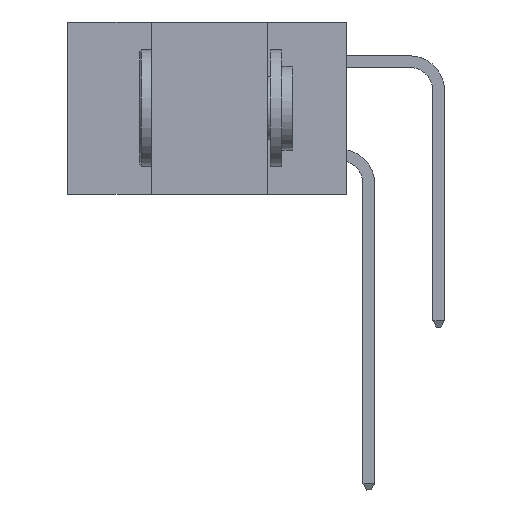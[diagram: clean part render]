
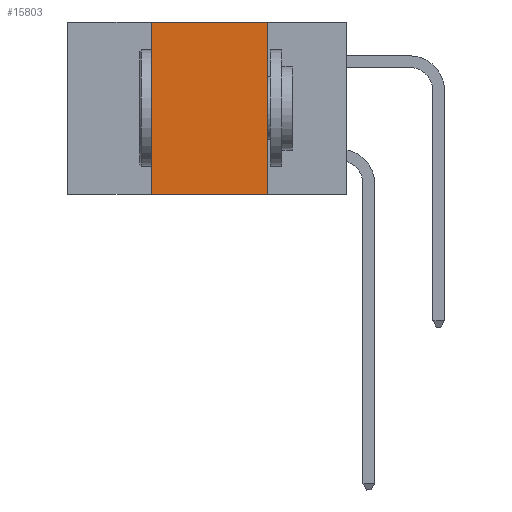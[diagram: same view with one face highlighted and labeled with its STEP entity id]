
A CAD part, left-side view. The second image highlights one B-rep face of the part: STEP entity #15803.
In plain terms, the highlighted planar face has unit normal (-1, 0, 0).
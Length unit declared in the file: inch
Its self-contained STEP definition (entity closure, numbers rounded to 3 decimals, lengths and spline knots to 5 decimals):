
#2 = VERTEX_POINT ( 'NONE', #9173 ) ;
#502 = CARTESIAN_POINT ( 'NONE',  ( 0., 0.6, 0. ) ) ;
#573 = VECTOR ( 'NONE', #6068, 39.37008 ) ;
#1725 = VECTOR ( 'NONE', #6852, 39.37008 ) ;
#2953 = CARTESIAN_POINT ( 'NONE',  ( 0., 0.6, -0.37 ) ) ;
#3042 = PLANE ( 'NONE',  #16402 ) ;
#3174 = EDGE_CURVE ( 'NONE', #15057, #2, #13434, .T. ) ;
#3556 = DIRECTION ( 'NONE',  ( 0., 0., 1. ) ) ;
#4239 = VERTEX_POINT ( 'NONE', #4954 ) ;
#4708 = LINE ( 'NONE', #2953, #1725 ) ;
#4954 = CARTESIAN_POINT ( 'NONE',  ( 0., 0.17, -0.37 ) ) ;
#5535 = DIRECTION ( 'NONE',  ( 0., 0., -1. ) ) ;
#5660 = ORIENTED_EDGE ( 'NONE', *, *, #14873, .F. ) ;
#6068 = DIRECTION ( 'NONE',  ( 0., -1., 0. ) ) ;
#6074 = CARTESIAN_POINT ( 'NONE',  ( 0., 0.42, 0. ) ) ;
#6337 = DIRECTION ( 'NONE',  ( 0., 0., -1. ) ) ;
#6374 = EDGE_CURVE ( 'NONE', #15057, #4239, #4708, .T. ) ;
#6852 = DIRECTION ( 'NONE',  ( 0., -1., 0. ) ) ;
#6942 = VERTEX_POINT ( 'NONE', #10939 ) ;
#7278 = VECTOR ( 'NONE', #6337, 39.37008 ) ;
#7786 = EDGE_LOOP ( 'NONE', ( #13539, #5660, #14173, #10088 ) ) ;
#8664 = LINE ( 'NONE', #15323, #7278 ) ;
#9173 = CARTESIAN_POINT ( 'NONE',  ( 0., 0.42, 0. ) ) ;
#9520 = DIRECTION ( 'NONE',  ( 1., 0., 0. ) ) ;
#9796 = FACE_OUTER_BOUND ( 'NONE', #7786, .T. ) ;
#10088 = ORIENTED_EDGE ( 'NONE', *, *, #6374, .T. ) ;
#10939 = CARTESIAN_POINT ( 'NONE',  ( 0., 0.17, 0. ) ) ;
#11497 = CARTESIAN_POINT ( 'NONE',  ( 0., 0.42, -0.37 ) ) ;
#11603 = LINE ( 'NONE', #15100, #573 ) ;
#12397 = EDGE_CURVE ( 'NONE', #6942, #4239, #8664, .T. ) ;
#13434 = LINE ( 'NONE', #6074, #16007 ) ;
#13539 = ORIENTED_EDGE ( 'NONE', *, *, #12397, .F. ) ;
#14173 = ORIENTED_EDGE ( 'NONE', *, *, #3174, .F. ) ;
#14873 = EDGE_CURVE ( 'NONE', #2, #6942, #11603, .T. ) ;
#15057 = VERTEX_POINT ( 'NONE', #11497 ) ;
#15100 = CARTESIAN_POINT ( 'NONE',  ( 0., 0.6, 0. ) ) ;
#15323 = CARTESIAN_POINT ( 'NONE',  ( 0., 0.17, 0. ) ) ;
#15803 = ADVANCED_FACE ( 'NONE', ( #9796 ), #3042, .F. ) ;
#16007 = VECTOR ( 'NONE', #3556, 39.37008 ) ;
#16402 = AXIS2_PLACEMENT_3D ( 'NONE', #502, #9520, #5535 ) ;
